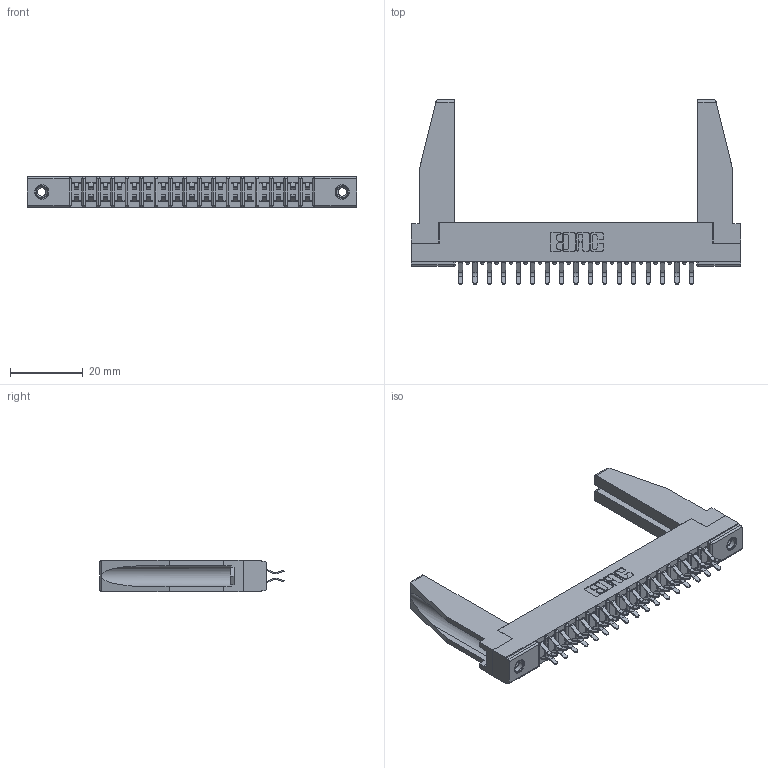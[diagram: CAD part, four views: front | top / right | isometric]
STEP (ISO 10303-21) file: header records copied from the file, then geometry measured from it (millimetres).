
FILE_DESCRIPTION (( 'STEP AP203' ), '1' );
FILE_NAME ('307-034-556-278.STEP', '2019-09-06T02:49:20', ( '' ), ( '' ), 'SwSTEP 2.0', 'SolidWorks 2016', '' );
FILE_SCHEMA (( 'CONFIG_CONTROL_DESIGN' ));
Length unit declared in the file: inch
Products named in the file (5): 345-250-001_345-250-001-102; 307-034-556-278; 307-220-078; 307-290-001_556; 307 Part_.156 Dia Mounting Holes
Assembly tree (39 placements, depth 2):
  307-034-556-278
    307 Part_.156 Dia Mounting Holes
    307-290-001_556  x34
    307-220-078  x2
    345-250-001_345-250-001-102  x2
Bounding box: 90.37 x 50.67 x 8.71 mm (x, y, z)
Volume: 9899.1 mm3; surface area: 13960.3 mm2
Topology: 39 solids, 39 shells, 1966 faces, 5481 edges, 3550 vertices
Faces by surface type: plane 1276, cylinder 638, sphere 36, cone 12, torus 4
Entity records: 20743 total; most frequent: CARTESIAN_POINT 3411, ORIENTED_EDGE 3336, DIRECTION 3306, EDGE_CURVE 1668, LINE 1272, VECTOR 1272, VERTEX_POINT 1080, AXIS2_PLACEMENT_3D 1017
